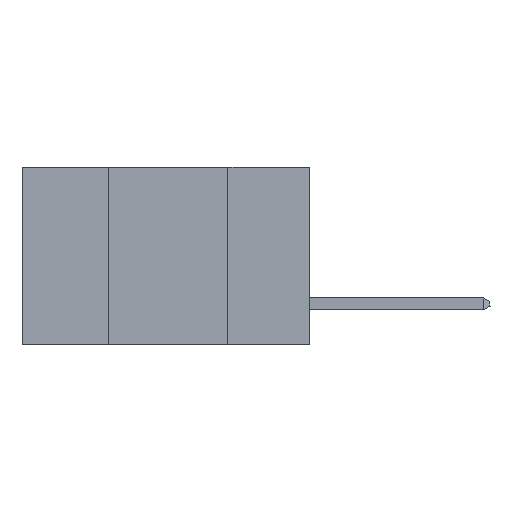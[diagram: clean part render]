
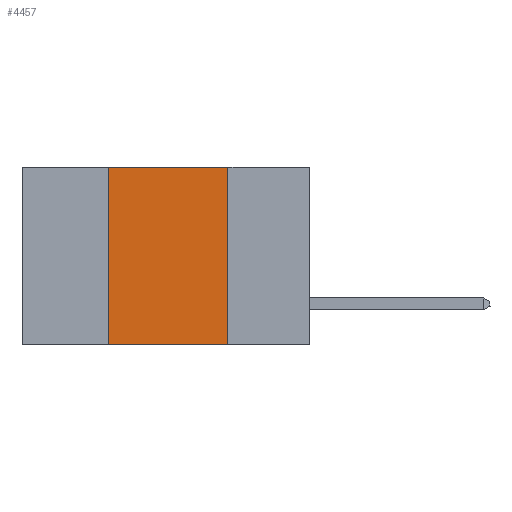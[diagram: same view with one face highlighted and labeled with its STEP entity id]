
A CAD part, left-side view. The second image highlights one B-rep face of the part: STEP entity #4457.
In plain terms, the highlighted planar face has unit normal (-1, 0, 0).
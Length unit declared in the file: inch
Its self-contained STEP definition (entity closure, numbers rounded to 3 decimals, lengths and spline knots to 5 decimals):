
#4457 = ADVANCED_FACE ( 'NONE', ( #10180 ), #11201, .F. ) ;
#4561 = DIRECTION ( 'NONE',  ( 0., -1., 0. ) ) ;
#5090 = LINE ( 'NONE', #8034, #13144 ) ;
#6034 = VERTEX_POINT ( 'NONE', #25605 ) ;
#7886 = LINE ( 'NONE', #14486, #30129 ) ;
#8034 = CARTESIAN_POINT ( 'NONE',  ( 0., 0.6, -0.37 ) ) ;
#9085 = DIRECTION ( 'NONE',  ( 1., 0., 0. ) ) ;
#9242 = CARTESIAN_POINT ( 'NONE',  ( 0., 0.42, 0. ) ) ;
#10180 = FACE_OUTER_BOUND ( 'NONE', #38802, .T. ) ;
#10475 = VECTOR ( 'NONE', #21987, 39.37008 ) ;
#11201 = PLANE ( 'NONE',  #20409 ) ;
#11589 = CARTESIAN_POINT ( 'NONE',  ( 0., 0.42, -0.37 ) ) ;
#12195 = CARTESIAN_POINT ( 'NONE',  ( 0., 0.6, 0. ) ) ;
#12740 = ORIENTED_EDGE ( 'NONE', *, *, #29758, .T. ) ;
#12780 = LINE ( 'NONE', #9242, #10475 ) ;
#12853 = CARTESIAN_POINT ( 'NONE',  ( 0., 0.17, -0.37 ) ) ;
#12906 = DIRECTION ( 'NONE',  ( 0., 0., -1. ) ) ;
#13144 = VECTOR ( 'NONE', #4561, 39.37008 ) ;
#14208 = VERTEX_POINT ( 'NONE', #12853 ) ;
#14486 = CARTESIAN_POINT ( 'NONE',  ( 0., 0.6, 0. ) ) ;
#18130 = VERTEX_POINT ( 'NONE', #26349 ) ;
#18774 = DIRECTION ( 'NONE',  ( 0., 0., -1. ) ) ;
#20409 = AXIS2_PLACEMENT_3D ( 'NONE', #12195, #9085, #12906 ) ;
#21115 = ORIENTED_EDGE ( 'NONE', *, *, #32977, .F. ) ;
#21200 = ORIENTED_EDGE ( 'NONE', *, *, #27639, .F. ) ;
#21987 = DIRECTION ( 'NONE',  ( 0., 0., 1. ) ) ;
#25605 = CARTESIAN_POINT ( 'NONE',  ( 0., 0.42, 0. ) ) ;
#25726 = VERTEX_POINT ( 'NONE', #11589 ) ;
#26349 = CARTESIAN_POINT ( 'NONE',  ( 0., 0.17, 0. ) ) ;
#27639 = EDGE_CURVE ( 'NONE', #6034, #18130, #7886, .T. ) ;
#28057 = LINE ( 'NONE', #33992, #33215 ) ;
#29758 = EDGE_CURVE ( 'NONE', #25726, #14208, #5090, .T. ) ;
#30129 = VECTOR ( 'NONE', #38658, 39.37008 ) ;
#32678 = ORIENTED_EDGE ( 'NONE', *, *, #34592, .F. ) ;
#32977 = EDGE_CURVE ( 'NONE', #18130, #14208, #28057, .T. ) ;
#33215 = VECTOR ( 'NONE', #18774, 39.37008 ) ;
#33992 = CARTESIAN_POINT ( 'NONE',  ( 0., 0.17, 0. ) ) ;
#34592 = EDGE_CURVE ( 'NONE', #25726, #6034, #12780, .T. ) ;
#38658 = DIRECTION ( 'NONE',  ( 0., -1., 0. ) ) ;
#38802 = EDGE_LOOP ( 'NONE', ( #21115, #21200, #32678, #12740 ) ) ;
